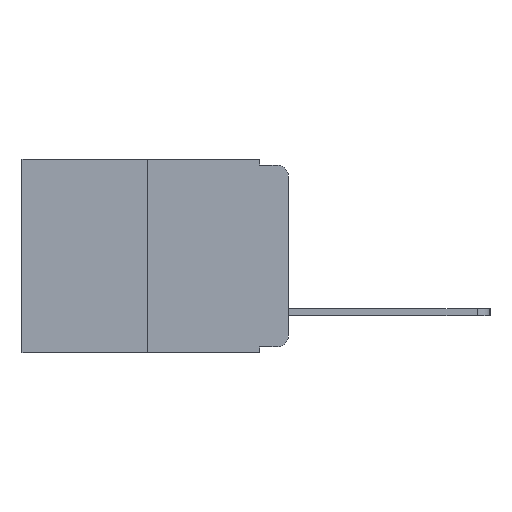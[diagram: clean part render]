
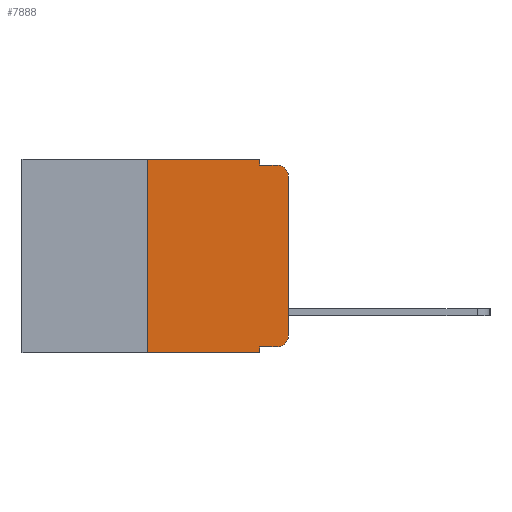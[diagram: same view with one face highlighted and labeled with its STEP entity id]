
A CAD part, left-side view. The second image highlights one B-rep face of the part: STEP entity #7888.
In plain terms, the highlighted planar face has unit normal (-1, 0, 0).
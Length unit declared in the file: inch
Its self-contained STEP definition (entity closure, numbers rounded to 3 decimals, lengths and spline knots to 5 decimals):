
#30 = EDGE_CURVE ( 'NONE', #6546, #1116, #6918, .T. ) ;
#137 = CARTESIAN_POINT ( 'NONE',  ( 0., 0.25, -0.343 ) ) ;
#149 = EDGE_CURVE ( 'NONE', #1901, #1116, #7541, .T. ) ;
#156 = LINE ( 'NONE', #3942, #9070 ) ;
#227 = ORIENTED_EDGE ( 'NONE', *, *, #149, .F. ) ;
#321 = VECTOR ( 'NONE', #10879, 39.37008 ) ;
#339 = EDGE_CURVE ( 'NONE', #4822, #1901, #156, .T. ) ;
#401 = VECTOR ( 'NONE', #1820, 39.37008 ) ;
#697 = EDGE_CURVE ( 'NONE', #4071, #7794, #6496, .T. ) ;
#759 = EDGE_CURVE ( 'NONE', #7220, #4715, #7410, .T. ) ;
#898 = EDGE_CURVE ( 'NONE', #7220, #2694, #9687, .T. ) ;
#925 = EDGE_CURVE ( 'NONE', #2694, #7701, #5022, .T. ) ;
#1025 = CARTESIAN_POINT ( 'NONE',  ( 0., 0.051, -0.01 ) ) ;
#1116 = VERTEX_POINT ( 'NONE', #6146 ) ;
#1127 = VECTOR ( 'NONE', #9321, 39.37008 ) ;
#1204 = ORIENTED_EDGE ( 'NONE', *, *, #6462, .F. ) ;
#1572 = CARTESIAN_POINT ( 'NONE',  ( 0., 0.02, -0.313 ) ) ;
#1578 = DIRECTION ( 'NONE',  ( -1., 0., 0. ) ) ;
#1754 = DIRECTION ( 'NONE',  ( 0., -1., 0. ) ) ;
#1820 = DIRECTION ( 'NONE',  ( 0., 0., 1. ) ) ;
#1901 = VERTEX_POINT ( 'NONE', #1025 ) ;
#1904 = LINE ( 'NONE', #3193, #8559 ) ;
#2031 = EDGE_CURVE ( 'NONE', #4071, #4715, #6868, .T. ) ;
#2216 = DIRECTION ( 'NONE',  ( 0., 0., -1. ) ) ;
#2316 = CARTESIAN_POINT ( 'NONE',  ( 0., 0.051, -0.333 ) ) ;
#2471 = CARTESIAN_POINT ( 'NONE',  ( 0., 0.051, -0.333 ) ) ;
#2568 = ORIENTED_EDGE ( 'NONE', *, *, #30, .T. ) ;
#2624 = DIRECTION ( 'NONE',  ( 0., 0., -1. ) ) ;
#2694 = VERTEX_POINT ( 'NONE', #9955 ) ;
#2786 = VECTOR ( 'NONE', #10017, 39.37008 ) ;
#2900 = CARTESIAN_POINT ( 'NONE',  ( 0., 0.051, 0. ) ) ;
#3193 = CARTESIAN_POINT ( 'NONE',  ( 0., 0.473, 0. ) ) ;
#3321 = LINE ( 'NONE', #8761, #401 ) ;
#3942 = CARTESIAN_POINT ( 'NONE',  ( 0., 0.051, 0. ) ) ;
#4048 = DIRECTION ( 'NONE',  ( 0., -1., 0. ) ) ;
#4071 = VERTEX_POINT ( 'NONE', #137 ) ;
#4279 = CARTESIAN_POINT ( 'NONE',  ( 0., 0.051, -0.01 ) ) ;
#4544 = AXIS2_PLACEMENT_3D ( 'NONE', #10852, #10639, #10624 ) ;
#4549 = ORIENTED_EDGE ( 'NONE', *, *, #759, .F. ) ;
#4715 = VERTEX_POINT ( 'NONE', #9042 ) ;
#4822 = VERTEX_POINT ( 'NONE', #10768 ) ;
#4922 = CARTESIAN_POINT ( 'NONE',  ( 0., 0.473, 0. ) ) ;
#5022 = CIRCLE ( 'NONE', #8413, 0.02 ) ;
#5518 = ORIENTED_EDGE ( 'NONE', *, *, #339, .F. ) ;
#5547 = CARTESIAN_POINT ( 'NONE',  ( 0., 0., -0.313 ) ) ;
#6146 = CARTESIAN_POINT ( 'NONE',  ( 0., 0.02, -0.01 ) ) ;
#6462 = EDGE_CURVE ( 'NONE', #7794, #4822, #1904, .T. ) ;
#6496 = LINE ( 'NONE', #9324, #1127 ) ;
#6546 = VERTEX_POINT ( 'NONE', #9988 ) ;
#6595 = VECTOR ( 'NONE', #10426, 39.37008 ) ;
#6868 = LINE ( 'NONE', #9136, #6595 ) ;
#6918 = CIRCLE ( 'NONE', #4544, 0.02 ) ;
#7220 = VERTEX_POINT ( 'NONE', #2316 ) ;
#7410 = LINE ( 'NONE', #2900, #2786 ) ;
#7480 = DIRECTION ( 'NONE',  ( 1., 0., 0. ) ) ;
#7524 = VECTOR ( 'NONE', #1754, 39.37008 ) ;
#7541 = LINE ( 'NONE', #4279, #321 ) ;
#7572 = AXIS2_PLACEMENT_3D ( 'NONE', #4922, #7480, #2216 ) ;
#7701 = VERTEX_POINT ( 'NONE', #5547 ) ;
#7794 = VERTEX_POINT ( 'NONE', #8973 ) ;
#7888 = ADVANCED_FACE ( 'NONE', ( #9678 ), #9849, .F. ) ;
#8229 = ORIENTED_EDGE ( 'NONE', *, *, #697, .F. ) ;
#8413 = AXIS2_PLACEMENT_3D ( 'NONE', #1572, #1578, #2624 ) ;
#8486 = ORIENTED_EDGE ( 'NONE', *, *, #2031, .T. ) ;
#8559 = VECTOR ( 'NONE', #4048, 39.37008 ) ;
#8761 = CARTESIAN_POINT ( 'NONE',  ( 0., 0., 0. ) ) ;
#8973 = CARTESIAN_POINT ( 'NONE',  ( 0., 0.25, 0. ) ) ;
#9012 = ORIENTED_EDGE ( 'NONE', *, *, #898, .T. ) ;
#9042 = CARTESIAN_POINT ( 'NONE',  ( 0., 0.051, -0.343 ) ) ;
#9070 = VECTOR ( 'NONE', #9368, 39.37008 ) ;
#9136 = CARTESIAN_POINT ( 'NONE',  ( 0., 0.473, -0.343 ) ) ;
#9318 = EDGE_CURVE ( 'NONE', #7701, #6546, #3321, .T. ) ;
#9321 = DIRECTION ( 'NONE',  ( 0., 0., 1. ) ) ;
#9324 = CARTESIAN_POINT ( 'NONE',  ( 0., 0.25, 0. ) ) ;
#9368 = DIRECTION ( 'NONE',  ( 0., 0., -1. ) ) ;
#9432 = EDGE_LOOP ( 'NONE', ( #11272, #2568, #227, #5518, #1204, #8229, #8486, #4549, #9012, #11155 ) ) ;
#9678 = FACE_OUTER_BOUND ( 'NONE', #9432, .T. ) ;
#9687 = LINE ( 'NONE', #2471, #7524 ) ;
#9849 = PLANE ( 'NONE',  #7572 ) ;
#9955 = CARTESIAN_POINT ( 'NONE',  ( 0., 0.02, -0.333 ) ) ;
#9988 = CARTESIAN_POINT ( 'NONE',  ( 0., 0., -0.03 ) ) ;
#10017 = DIRECTION ( 'NONE',  ( 0., 0., -1. ) ) ;
#10426 = DIRECTION ( 'NONE',  ( 0., -1., 0. ) ) ;
#10624 = DIRECTION ( 'NONE',  ( 0., 0., -1. ) ) ;
#10639 = DIRECTION ( 'NONE',  ( -1., 0., 0. ) ) ;
#10768 = CARTESIAN_POINT ( 'NONE',  ( 0., 0.051, 0. ) ) ;
#10852 = CARTESIAN_POINT ( 'NONE',  ( 0., 0.02, -0.03 ) ) ;
#10879 = DIRECTION ( 'NONE',  ( 0., -1., 0. ) ) ;
#11155 = ORIENTED_EDGE ( 'NONE', *, *, #925, .T. ) ;
#11272 = ORIENTED_EDGE ( 'NONE', *, *, #9318, .T. ) ;
